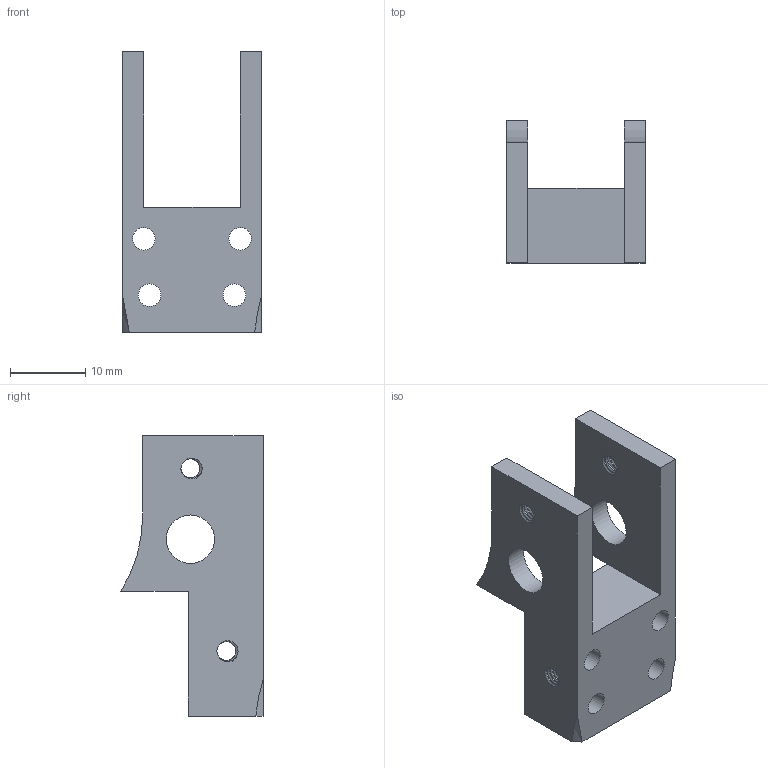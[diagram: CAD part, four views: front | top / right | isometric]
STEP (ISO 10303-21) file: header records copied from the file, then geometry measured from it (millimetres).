
FILE_DESCRIPTION(/* description */ (''),/* implementation_level */ '2;1');
FILE_NAME(/* name */ 'GG Buffer Mount.step',/* time_stamp */ '2024-01-16T15:54:55-05:00',/* author */ (''),/* organization */ (''),/* preprocessor_version */ 'ST-DEVELOPER v20',/* originating_system */ 'Autodesk Translation Framework v12.14.0.127',/* authorisation */ '');
FILE_SCHEMA (('AUTOMOTIVE_DESIGN { 1 0 10303 214 3 1 1 }'));
Length unit declared in the file: inch
Products named in the file (1): GG Buffer Mount
Bounding box: 18.44 x 18.89 x 37.21 mm (x, y, z)
Volume: 4348.5 mm3; surface area: 3595 mm2
Topology: 1 solids, 1 shells, 134 faces, 394 edges, 262 vertices
Faces by surface type: cylinder 112, plane 14, bspline 8
Full cylindrical faces by diameter (mm): 2.529 x24, 3 x4, 3.086 x14, 6.426 x2
Entity records: 10177 total; most frequent: CARTESIAN_POINT 6960, ORIENTED_EDGE 788, DIRECTION 462, EDGE_CURVE 394, VERTEX_POINT 262, B_SPLINE_CURVE_WITH_KNOTS 220, AXIS2_PLACEMENT_3D 161, EDGE_LOOP 152
